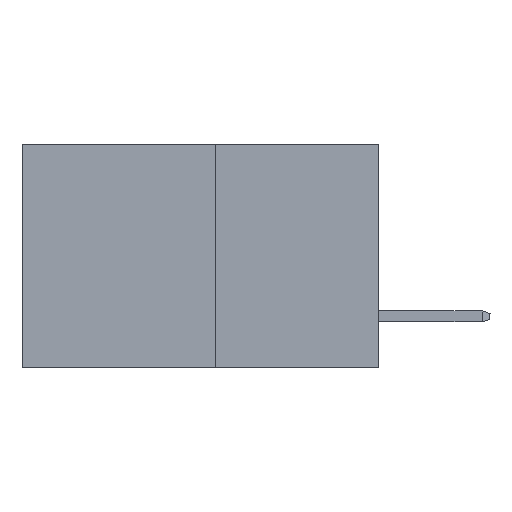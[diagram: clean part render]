
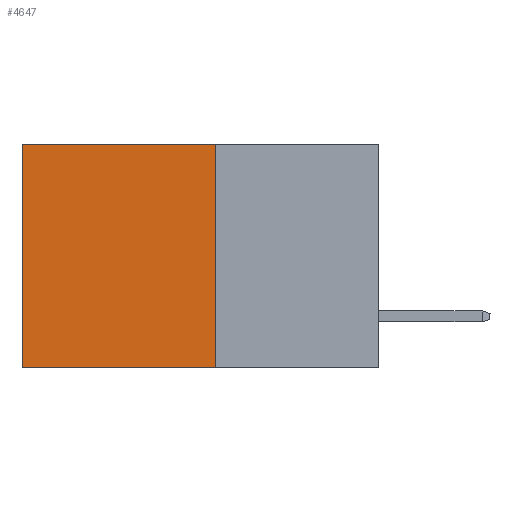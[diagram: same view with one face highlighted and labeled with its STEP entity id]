
A CAD part, left-side view. The second image highlights one B-rep face of the part: STEP entity #4647.
In plain terms, the highlighted planar face has unit normal (-1, 0, 0).
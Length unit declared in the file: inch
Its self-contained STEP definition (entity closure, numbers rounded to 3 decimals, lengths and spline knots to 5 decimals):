
#183 = DIRECTION ( 'NONE',  ( 0., 1., 0. ) ) ;
#286 = DIRECTION ( 'NONE',  ( 0., 0., -1. ) ) ;
#1217 = LINE ( 'NONE', #1905, #2871 ) ;
#1343 = VERTEX_POINT ( 'NONE', #10012 ) ;
#1735 = VECTOR ( 'NONE', #183, 39.37008 ) ;
#1905 = CARTESIAN_POINT ( 'NONE',  ( 0.277, 0.27, -0.37 ) ) ;
#2337 = ORIENTED_EDGE ( 'NONE', *, *, #8001, .F. ) ;
#2361 = EDGE_LOOP ( 'NONE', ( #8272, #4136, #2337, #8973 ) ) ;
#2812 = VERTEX_POINT ( 'NONE', #6764 ) ;
#2871 = VECTOR ( 'NONE', #286, 39.37008 ) ;
#2920 = CARTESIAN_POINT ( 'NONE',  ( 0.277, 0.59, -0.37 ) ) ;
#2954 = DIRECTION ( 'NONE',  ( 0., 0., -1. ) ) ;
#3169 = VECTOR ( 'NONE', #9842, 39.37008 ) ;
#3770 = DIRECTION ( 'NONE',  ( 0., 0., -1. ) ) ;
#3772 = DIRECTION ( 'NONE',  ( 1., 0., 0. ) ) ;
#3794 = PLANE ( 'NONE',  #7789 ) ;
#3906 = CARTESIAN_POINT ( 'NONE',  ( 0.277, 0.27, -0.37 ) ) ;
#4136 = ORIENTED_EDGE ( 'NONE', *, *, #7880, .F. ) ;
#4332 = LINE ( 'NONE', #4441, #1735 ) ;
#4441 = CARTESIAN_POINT ( 'NONE',  ( 0.277, 0.27, -0.37 ) ) ;
#4528 = VERTEX_POINT ( 'NONE', #5693 ) ;
#4647 = ADVANCED_FACE ( 'NONE', ( #8096 ), #3794, .F. ) ;
#4931 = VERTEX_POINT ( 'NONE', #10172 ) ;
#5559 = LINE ( 'NONE', #8322, #3169 ) ;
#5693 = CARTESIAN_POINT ( 'NONE',  ( 0.277, 0.59, -0.37 ) ) ;
#6077 = EDGE_CURVE ( 'NONE', #2812, #4931, #5559, .T. ) ;
#6429 = VECTOR ( 'NONE', #2954, 39.37008 ) ;
#6480 = EDGE_CURVE ( 'NONE', #4931, #4528, #6970, .T. ) ;
#6764 = CARTESIAN_POINT ( 'NONE',  ( 0.277, 0.27, 0. ) ) ;
#6970 = LINE ( 'NONE', #2920, #6429 ) ;
#7789 = AXIS2_PLACEMENT_3D ( 'NONE', #3906, #3772, #3770 ) ;
#7880 = EDGE_CURVE ( 'NONE', #1343, #4528, #4332, .T. ) ;
#8001 = EDGE_CURVE ( 'NONE', #2812, #1343, #1217, .T. ) ;
#8096 = FACE_OUTER_BOUND ( 'NONE', #2361, .T. ) ;
#8272 = ORIENTED_EDGE ( 'NONE', *, *, #6480, .T. ) ;
#8322 = CARTESIAN_POINT ( 'NONE',  ( 0.277, 0.27, 0. ) ) ;
#8973 = ORIENTED_EDGE ( 'NONE', *, *, #6077, .T. ) ;
#9842 = DIRECTION ( 'NONE',  ( 0., 1., 0. ) ) ;
#10012 = CARTESIAN_POINT ( 'NONE',  ( 0.277, 0.27, -0.37 ) ) ;
#10172 = CARTESIAN_POINT ( 'NONE',  ( 0.277, 0.59, 0. ) ) ;
